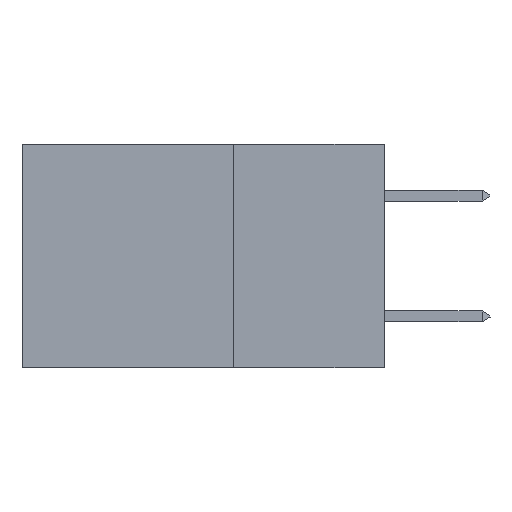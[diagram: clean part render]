
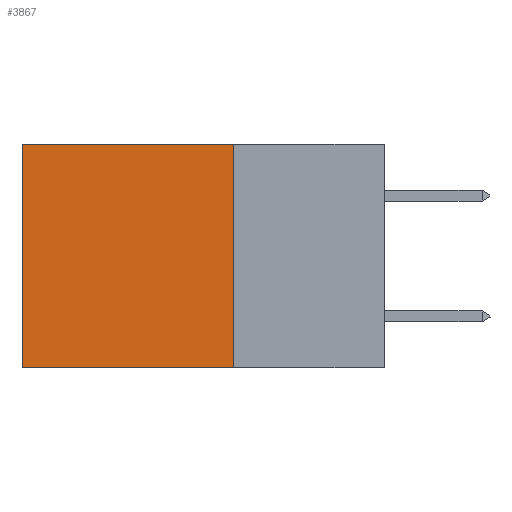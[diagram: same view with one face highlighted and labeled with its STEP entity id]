
A CAD part, left-side view. The second image highlights one B-rep face of the part: STEP entity #3867.
In plain terms, the highlighted planar face has unit normal (-1, 0, 0).
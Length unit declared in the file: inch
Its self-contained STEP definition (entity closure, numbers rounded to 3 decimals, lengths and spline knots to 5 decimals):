
#385 = DIRECTION ( 'NONE',  ( 0., 0., -1. ) ) ;
#1086 = DIRECTION ( 'NONE',  ( 0., 0., -1. ) ) ;
#1180 = CARTESIAN_POINT ( 'NONE',  ( 0.2875, 0.6, 0. ) ) ;
#1276 = ORIENTED_EDGE ( 'NONE', *, *, #4513, .F. ) ;
#1507 = VERTEX_POINT ( 'NONE', #9209 ) ;
#1594 = EDGE_CURVE ( 'NONE', #9801, #5929, #4969, .T. ) ;
#1801 = FACE_OUTER_BOUND ( 'NONE', #12886, .T. ) ;
#1879 = ORIENTED_EDGE ( 'NONE', *, *, #10647, .T. ) ;
#3110 = CARTESIAN_POINT ( 'NONE',  ( 0.2875, 0.25, -0.37 ) ) ;
#3435 = AXIS2_PLACEMENT_3D ( 'NONE', #5570, #6614, #385 ) ;
#3867 = ADVANCED_FACE ( 'NONE', ( #1801 ), #10341, .F. ) ;
#3974 = DIRECTION ( 'NONE',  ( 0., 1., 0. ) ) ;
#4059 = DIRECTION ( 'NONE',  ( 0., 0., -1. ) ) ;
#4513 = EDGE_CURVE ( 'NONE', #1507, #13164, #6321, .T. ) ;
#4544 = CARTESIAN_POINT ( 'NONE',  ( 0.2875, 0.25, -0.37 ) ) ;
#4969 = LINE ( 'NONE', #1180, #5625 ) ;
#5570 = CARTESIAN_POINT ( 'NONE',  ( 0.2875, 0.25, 0. ) ) ;
#5625 = VECTOR ( 'NONE', #1086, 39.37008 ) ;
#5929 = VERTEX_POINT ( 'NONE', #12080 ) ;
#6321 = LINE ( 'NONE', #9986, #7294 ) ;
#6607 = ORIENTED_EDGE ( 'NONE', *, *, #6900, .F. ) ;
#6614 = DIRECTION ( 'NONE',  ( 1., 0., 0. ) ) ;
#6900 = EDGE_CURVE ( 'NONE', #13164, #5929, #12440, .T. ) ;
#7294 = VECTOR ( 'NONE', #4059, 39.37008 ) ;
#7651 = ORIENTED_EDGE ( 'NONE', *, *, #1594, .T. ) ;
#9137 = CARTESIAN_POINT ( 'NONE',  ( 0.2875, 0.25, 0. ) ) ;
#9209 = CARTESIAN_POINT ( 'NONE',  ( 0.2875, 0.25, 0. ) ) ;
#9801 = VERTEX_POINT ( 'NONE', #13220 ) ;
#9986 = CARTESIAN_POINT ( 'NONE',  ( 0.2875, 0.25, 0. ) ) ;
#10341 = PLANE ( 'NONE',  #3435 ) ;
#10412 = LINE ( 'NONE', #9137, #12843 ) ;
#10647 = EDGE_CURVE ( 'NONE', #1507, #9801, #10412, .T. ) ;
#11559 = DIRECTION ( 'NONE',  ( 0., 1., 0. ) ) ;
#11821 = VECTOR ( 'NONE', #11559, 39.37008 ) ;
#12080 = CARTESIAN_POINT ( 'NONE',  ( 0.2875, 0.6, -0.37 ) ) ;
#12440 = LINE ( 'NONE', #3110, #11821 ) ;
#12843 = VECTOR ( 'NONE', #3974, 39.37008 ) ;
#12886 = EDGE_LOOP ( 'NONE', ( #7651, #6607, #1276, #1879 ) ) ;
#13164 = VERTEX_POINT ( 'NONE', #4544 ) ;
#13220 = CARTESIAN_POINT ( 'NONE',  ( 0.2875, 0.6, 0. ) ) ;
